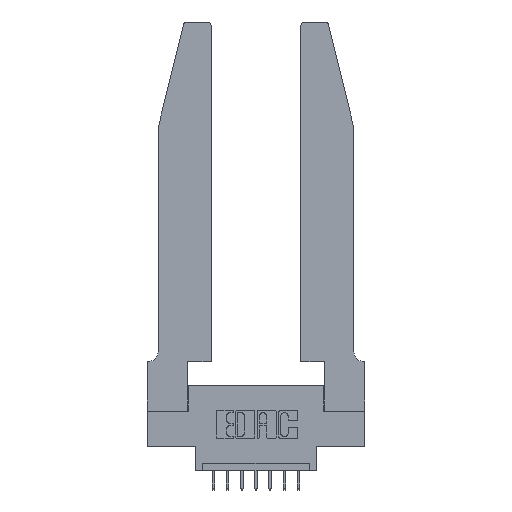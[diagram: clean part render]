
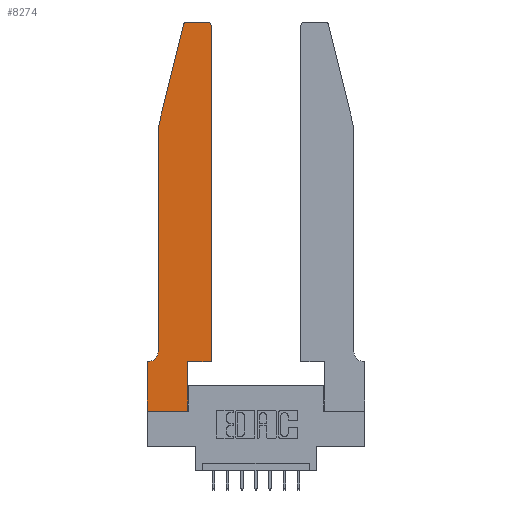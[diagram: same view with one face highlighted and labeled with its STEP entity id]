
A CAD part, top view. The second image highlights one B-rep face of the part: STEP entity #8274.
In plain terms, the highlighted planar face has unit normal (0, 0, 1).
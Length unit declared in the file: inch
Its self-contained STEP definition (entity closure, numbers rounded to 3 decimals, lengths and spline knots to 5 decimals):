
#34 = EDGE_CURVE ( 'NONE', #7735, #5943, #3017, .T. ) ;
#343 = LINE ( 'NONE', #4966, #5377 ) ;
#485 = DIRECTION ( 'NONE',  ( 0., 0., 1. ) ) ;
#724 = VERTEX_POINT ( 'NONE', #1797 ) ;
#756 = ORIENTED_EDGE ( 'NONE', *, *, #11587, .T. ) ;
#843 = CARTESIAN_POINT ( 'NONE',  ( 0.0055, 0.35, 0.37 ) ) ;
#1031 = CARTESIAN_POINT ( 'NONE',  ( 0.0755, 2., 0.37 ) ) ;
#1074 = CARTESIAN_POINT ( 'NONE',  ( 0., 0., 0.37 ) ) ;
#1156 = AXIS2_PLACEMENT_3D ( 'NONE', #13282, #1646, #5200 ) ;
#1319 = CARTESIAN_POINT ( 'NONE',  ( 0.0755, 0.42, 0.37 ) ) ;
#1512 = ORIENTED_EDGE ( 'NONE', *, *, #12973, .T. ) ;
#1543 = DIRECTION ( 'NONE',  ( -1., 0., 0. ) ) ;
#1619 = CARTESIAN_POINT ( 'NONE',  ( 0.284, 2.72, 0.37 ) ) ;
#1646 = DIRECTION ( 'NONE',  ( 0., 0., 1. ) ) ;
#1797 = CARTESIAN_POINT ( 'NONE',  ( 0.284, 2.75, 0.37 ) ) ;
#1874 = ORIENTED_EDGE ( 'NONE', *, *, #10963, .T. ) ;
#1892 = VECTOR ( 'NONE', #5729, 39.37008 ) ;
#2003 = LINE ( 'NONE', #1074, #6247 ) ;
#2010 = EDGE_CURVE ( 'NONE', #13905, #8741, #343, .T. ) ;
#2095 = ORIENTED_EDGE ( 'NONE', *, *, #34, .T. ) ;
#2146 = VECTOR ( 'NONE', #9783, 39.37008 ) ;
#2375 = AXIS2_PLACEMENT_3D ( 'NONE', #10018, #14626, #4273 ) ;
#2650 = VECTOR ( 'NONE', #14268, 39.37008 ) ;
#2701 = LINE ( 'NONE', #5182, #9160 ) ;
#2924 = ORIENTED_EDGE ( 'NONE', *, *, #13727, .T. ) ;
#2948 = ORIENTED_EDGE ( 'NONE', *, *, #12964, .T. ) ;
#3017 = LINE ( 'NONE', #8899, #10897 ) ;
#3022 = VECTOR ( 'NONE', #5773, 39.37008 ) ;
#3669 = DIRECTION ( 'NONE',  ( 1., 0., 0. ) ) ;
#3876 = VERTEX_POINT ( 'NONE', #5324 ) ;
#4273 = DIRECTION ( 'NONE',  ( -1., 0., 0. ) ) ;
#4368 = CARTESIAN_POINT ( 'NONE',  ( 0.4505, 2.72, 0.37 ) ) ;
#4514 = AXIS2_PLACEMENT_3D ( 'NONE', #11076, #7747, #14415 ) ;
#4656 = EDGE_CURVE ( 'NONE', #14066, #13905, #10533, .T. ) ;
#4966 = CARTESIAN_POINT ( 'NONE',  ( 0.4505, 0.35, 0.37 ) ) ;
#5182 = CARTESIAN_POINT ( 'NONE',  ( 0.2605, 2.75, 0.37 ) ) ;
#5200 = DIRECTION ( 'NONE',  ( 1., 0., 0. ) ) ;
#5324 = CARTESIAN_POINT ( 'NONE',  ( 0., 0., 0.37 ) ) ;
#5376 = ORIENTED_EDGE ( 'NONE', *, *, #4656, .T. ) ;
#5377 = VECTOR ( 'NONE', #14180, 39.37008 ) ;
#5641 = DIRECTION ( 'NONE',  ( 0., 1., 0. ) ) ;
#5698 = DIRECTION ( 'NONE',  ( 0., -1., 0. ) ) ;
#5729 = DIRECTION ( 'NONE',  ( 0., -1., 0. ) ) ;
#5773 = DIRECTION ( 'NONE',  ( 0., 1., 0. ) ) ;
#5943 = VERTEX_POINT ( 'NONE', #7905 ) ;
#6247 = VECTOR ( 'NONE', #5698, 39.37008 ) ;
#6274 = CIRCLE ( 'NONE', #8178, 0.03 ) ;
#6352 = VERTEX_POINT ( 'NONE', #7346 ) ;
#6471 = CIRCLE ( 'NONE', #2375, 0.07 ) ;
#6473 = ORIENTED_EDGE ( 'NONE', *, *, #14316, .T. ) ;
#6501 = VECTOR ( 'NONE', #5641, 39.37008 ) ;
#6548 = FACE_OUTER_BOUND ( 'NONE', #13702, .T. ) ;
#6556 = LINE ( 'NONE', #13210, #2650 ) ;
#6757 = CARTESIAN_POINT ( 'NONE',  ( 0.4505, 0.35, 0.37 ) ) ;
#7084 = CARTESIAN_POINT ( 'NONE',  ( 0.4205, 2.75, 0.37 ) ) ;
#7148 = ORIENTED_EDGE ( 'NONE', *, *, #2010, .T. ) ;
#7250 = VERTEX_POINT ( 'NONE', #1319 ) ;
#7346 = CARTESIAN_POINT ( 'NONE',  ( 0.0755, 2., 0.37 ) ) ;
#7735 = VERTEX_POINT ( 'NONE', #843 ) ;
#7747 = DIRECTION ( 'NONE',  ( 0., 0., 1. ) ) ;
#7757 = LINE ( 'NONE', #10112, #6501 ) ;
#7905 = CARTESIAN_POINT ( 'NONE',  ( 0., 0.35, 0.37 ) ) ;
#8158 = VERTEX_POINT ( 'NONE', #7084 ) ;
#8178 = AXIS2_PLACEMENT_3D ( 'NONE', #1619, #485, #3669 ) ;
#8244 = VERTEX_POINT ( 'NONE', #12297 ) ;
#8274 = ADVANCED_FACE ( 'NONE', ( #6548 ), #11149, .T. ) ;
#8741 = VERTEX_POINT ( 'NONE', #6757 ) ;
#8899 = CARTESIAN_POINT ( 'NONE',  ( 0.0755, 0.35, 0.37 ) ) ;
#8912 = LINE ( 'NONE', #14384, #2146 ) ;
#9160 = VECTOR ( 'NONE', #1543, 39.37008 ) ;
#9181 = ORIENTED_EDGE ( 'NONE', *, *, #13347, .T. ) ;
#9277 = VERTEX_POINT ( 'NONE', #4368 ) ;
#9751 = DIRECTION ( 'NONE',  ( -1., 0., 0. ) ) ;
#9767 = EDGE_CURVE ( 'NONE', #7250, #7735, #6471, .T. ) ;
#9783 = DIRECTION ( 'NONE',  ( 1., 0., 0. ) ) ;
#9893 = CIRCLE ( 'NONE', #1156, 0.03 ) ;
#10018 = CARTESIAN_POINT ( 'NONE',  ( 0.0055, 0.42, 0.37 ) ) ;
#10112 = CARTESIAN_POINT ( 'NONE',  ( 0.4505, 0.35, 0.37 ) ) ;
#10309 = CARTESIAN_POINT ( 'NONE',  ( 0.2865, 0.35, 0.37 ) ) ;
#10426 = EDGE_CURVE ( 'NONE', #6352, #7250, #11400, .T. ) ;
#10533 = LINE ( 'NONE', #10309, #3022 ) ;
#10691 = ORIENTED_EDGE ( 'NONE', *, *, #10426, .T. ) ;
#10897 = VECTOR ( 'NONE', #9751, 39.37008 ) ;
#10963 = EDGE_CURVE ( 'NONE', #5943, #3876, #2003, .T. ) ;
#11076 = CARTESIAN_POINT ( 'NONE',  ( 0., 0.35, 0.37 ) ) ;
#11149 = PLANE ( 'NONE',  #4514 ) ;
#11400 = LINE ( 'NONE', #1031, #1892 ) ;
#11484 = CARTESIAN_POINT ( 'NONE',  ( 0.2865, 0.35, 0.37 ) ) ;
#11587 = EDGE_CURVE ( 'NONE', #724, #8244, #6274, .T. ) ;
#11939 = CARTESIAN_POINT ( 'NONE',  ( 0.2865, 0., 0.37 ) ) ;
#12297 = CARTESIAN_POINT ( 'NONE',  ( 0.25487, 2.72718, 0.37 ) ) ;
#12964 = EDGE_CURVE ( 'NONE', #9277, #8158, #9893, .T. ) ;
#12973 = EDGE_CURVE ( 'NONE', #8244, #6352, #6556, .T. ) ;
#13210 = CARTESIAN_POINT ( 'NONE',  ( 0.0755, 2., 0.37 ) ) ;
#13282 = CARTESIAN_POINT ( 'NONE',  ( 0.4205, 2.72, 0.37 ) ) ;
#13347 = EDGE_CURVE ( 'NONE', #8158, #724, #2701, .T. ) ;
#13702 = EDGE_LOOP ( 'NONE', ( #9181, #756, #1512, #10691, #13772, #2095, #1874, #2924, #5376, #7148, #6473, #2948 ) ) ;
#13727 = EDGE_CURVE ( 'NONE', #3876, #14066, #8912, .T. ) ;
#13772 = ORIENTED_EDGE ( 'NONE', *, *, #9767, .T. ) ;
#13905 = VERTEX_POINT ( 'NONE', #11484 ) ;
#14066 = VERTEX_POINT ( 'NONE', #11939 ) ;
#14180 = DIRECTION ( 'NONE',  ( 1., 0., 0. ) ) ;
#14268 = DIRECTION ( 'NONE',  ( -0.239, -0.971, 0. ) ) ;
#14316 = EDGE_CURVE ( 'NONE', #8741, #9277, #7757, .T. ) ;
#14384 = CARTESIAN_POINT ( 'NONE',  ( 0., 0., 0.37 ) ) ;
#14415 = DIRECTION ( 'NONE',  ( 1., 0., 0. ) ) ;
#14626 = DIRECTION ( 'NONE',  ( 0., 0., -1. ) ) ;
